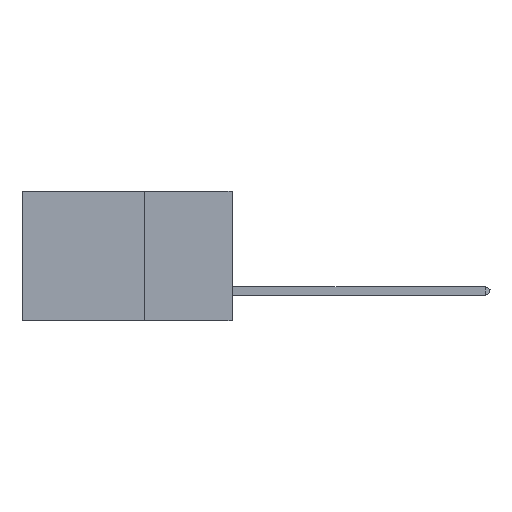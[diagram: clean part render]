
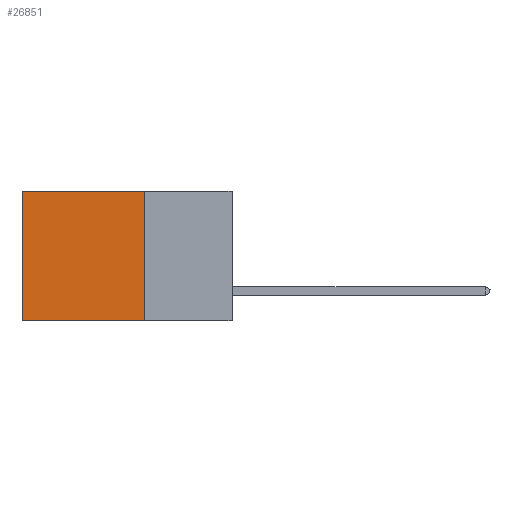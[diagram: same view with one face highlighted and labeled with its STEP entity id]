
A CAD part, left-side view. The second image highlights one B-rep face of the part: STEP entity #26851.
In plain terms, the highlighted planar face has unit normal (-1, 0, 0).
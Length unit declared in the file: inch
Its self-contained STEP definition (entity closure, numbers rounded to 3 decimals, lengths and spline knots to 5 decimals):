
#1485 = EDGE_CURVE ( 'NONE', #2742, #3473, #11800, .T. ) ;
#2742 = VERTEX_POINT ( 'NONE', #13603 ) ;
#2802 = VERTEX_POINT ( 'NONE', #15985 ) ;
#3473 = VERTEX_POINT ( 'NONE', #8663 ) ;
#4505 = VECTOR ( 'NONE', #17610, 39.37008 ) ;
#5608 = CARTESIAN_POINT ( 'NONE',  ( 0.2875, 0.25, 0. ) ) ;
#5914 = CARTESIAN_POINT ( 'NONE',  ( 0.2875, 0.25, 0. ) ) ;
#6967 = DIRECTION ( 'NONE',  ( 0., 0., -1. ) ) ;
#8663 = CARTESIAN_POINT ( 'NONE',  ( 0.2875, 0.6, -0.37 ) ) ;
#9327 = DIRECTION ( 'NONE',  ( 0., 1., 0. ) ) ;
#9712 = DIRECTION ( 'NONE',  ( 0., 1., 0. ) ) ;
#9792 = ORIENTED_EDGE ( 'NONE', *, *, #26175, .F. ) ;
#10495 = VECTOR ( 'NONE', #20816, 39.37008 ) ;
#10598 = LINE ( 'NONE', #19968, #16930 ) ;
#11065 = DIRECTION ( 'NONE',  ( 1., 0., 0. ) ) ;
#11365 = ORIENTED_EDGE ( 'NONE', *, *, #24628, .F. ) ;
#11645 = VERTEX_POINT ( 'NONE', #5608 ) ;
#11800 = LINE ( 'NONE', #26209, #4505 ) ;
#13603 = CARTESIAN_POINT ( 'NONE',  ( 0.2875, 0.6, 0. ) ) ;
#15354 = CARTESIAN_POINT ( 'NONE',  ( 0.2875, 0.25, 0. ) ) ;
#15723 = EDGE_CURVE ( 'NONE', #11645, #2742, #18527, .T. ) ;
#15737 = AXIS2_PLACEMENT_3D ( 'NONE', #15354, #11065, #6967 ) ;
#15985 = CARTESIAN_POINT ( 'NONE',  ( 0.2875, 0.25, -0.37 ) ) ;
#16930 = VECTOR ( 'NONE', #9327, 39.37008 ) ;
#17610 = DIRECTION ( 'NONE',  ( 0., 0., -1. ) ) ;
#18262 = ORIENTED_EDGE ( 'NONE', *, *, #15723, .T. ) ;
#18527 = LINE ( 'NONE', #22523, #25564 ) ;
#19158 = FACE_OUTER_BOUND ( 'NONE', #23334, .T. ) ;
#19754 = PLANE ( 'NONE',  #15737 ) ;
#19968 = CARTESIAN_POINT ( 'NONE',  ( 0.2875, 0.25, -0.37 ) ) ;
#20816 = DIRECTION ( 'NONE',  ( 0., 0., -1. ) ) ;
#22523 = CARTESIAN_POINT ( 'NONE',  ( 0.2875, 0.25, 0. ) ) ;
#23334 = EDGE_LOOP ( 'NONE', ( #27530, #11365, #9792, #18262 ) ) ;
#24628 = EDGE_CURVE ( 'NONE', #2802, #3473, #10598, .T. ) ;
#25564 = VECTOR ( 'NONE', #9712, 39.37008 ) ;
#26175 = EDGE_CURVE ( 'NONE', #11645, #2802, #27213, .T. ) ;
#26209 = CARTESIAN_POINT ( 'NONE',  ( 0.2875, 0.6, 0. ) ) ;
#26851 = ADVANCED_FACE ( 'NONE', ( #19158 ), #19754, .F. ) ;
#27213 = LINE ( 'NONE', #5914, #10495 ) ;
#27530 = ORIENTED_EDGE ( 'NONE', *, *, #1485, .T. ) ;
